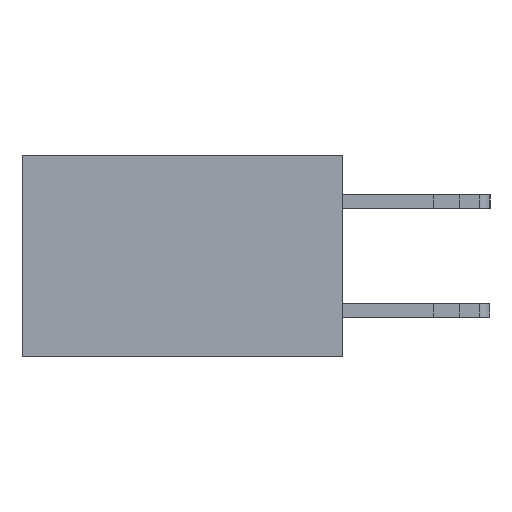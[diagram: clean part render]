
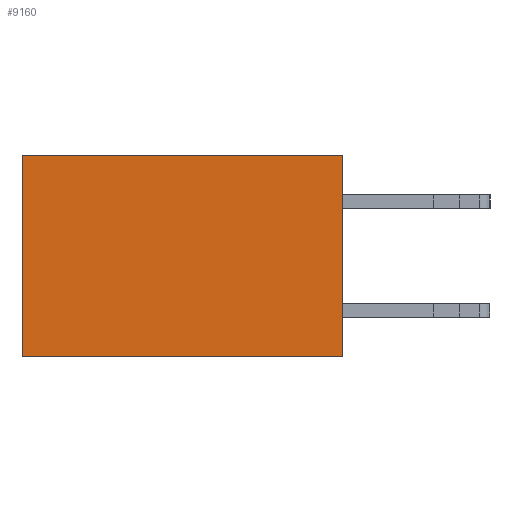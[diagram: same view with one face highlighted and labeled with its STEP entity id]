
A CAD part, left-side view. The second image highlights one B-rep face of the part: STEP entity #9160.
In plain terms, the highlighted planar face has unit normal (-1, 0, 0).
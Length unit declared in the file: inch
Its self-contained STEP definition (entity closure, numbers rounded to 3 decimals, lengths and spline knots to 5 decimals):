
#877 = VERTEX_POINT ( 'NONE', #22415 ) ;
#1611 = ORIENTED_EDGE ( 'NONE', *, *, #1914, .T. ) ;
#1914 = EDGE_CURVE ( 'NONE', #23389, #8918, #18854, .T. ) ;
#2742 = CARTESIAN_POINT ( 'NONE',  ( 0.277, 0., -0.37 ) ) ;
#3671 = DIRECTION ( 'NONE',  ( 0., 0., -1. ) ) ;
#3804 = VECTOR ( 'NONE', #12381, 39.37008 ) ;
#4152 = CARTESIAN_POINT ( 'NONE',  ( 0.277, 0., -0.37 ) ) ;
#6140 = DIRECTION ( 'NONE',  ( 0., 1., 0. ) ) ;
#6161 = VERTEX_POINT ( 'NONE', #11877 ) ;
#6810 = EDGE_LOOP ( 'NONE', ( #1611, #12000, #22275, #7375 ) ) ;
#7375 = ORIENTED_EDGE ( 'NONE', *, *, #15872, .T. ) ;
#7888 = DIRECTION ( 'NONE',  ( 0., 0., -1. ) ) ;
#8499 = VECTOR ( 'NONE', #7888, 39.37008 ) ;
#8918 = VERTEX_POINT ( 'NONE', #22404 ) ;
#9160 = ADVANCED_FACE ( 'NONE', ( #15020 ), #15302, .F. ) ;
#9585 = LINE ( 'NONE', #2742, #19305 ) ;
#9665 = VECTOR ( 'NONE', #6140, 39.37008 ) ;
#10373 = CARTESIAN_POINT ( 'NONE',  ( 0.277, 0., 0. ) ) ;
#11195 = EDGE_CURVE ( 'NONE', #6161, #877, #9585, .T. ) ;
#11877 = CARTESIAN_POINT ( 'NONE',  ( 0.277, 0., 0. ) ) ;
#12000 = ORIENTED_EDGE ( 'NONE', *, *, #19004, .F. ) ;
#12381 = DIRECTION ( 'NONE',  ( 0., 1., 0. ) ) ;
#13451 = CARTESIAN_POINT ( 'NONE',  ( 0.277, 0., -0.37 ) ) ;
#14214 = LINE ( 'NONE', #10373, #3804 ) ;
#14872 = LINE ( 'NONE', #4152, #9665 ) ;
#15020 = FACE_OUTER_BOUND ( 'NONE', #6810, .T. ) ;
#15302 = PLANE ( 'NONE',  #22919 ) ;
#15387 = DIRECTION ( 'NONE',  ( 1., 0., 0. ) ) ;
#15872 = EDGE_CURVE ( 'NONE', #6161, #23389, #14214, .T. ) ;
#16407 = DIRECTION ( 'NONE',  ( 0., 0., -1. ) ) ;
#16441 = CARTESIAN_POINT ( 'NONE',  ( 0.277, 0.59, 0. ) ) ;
#18854 = LINE ( 'NONE', #22325, #8499 ) ;
#19004 = EDGE_CURVE ( 'NONE', #877, #8918, #14872, .T. ) ;
#19305 = VECTOR ( 'NONE', #16407, 39.37008 ) ;
#22275 = ORIENTED_EDGE ( 'NONE', *, *, #11195, .F. ) ;
#22325 = CARTESIAN_POINT ( 'NONE',  ( 0.277, 0.59, -0.37 ) ) ;
#22404 = CARTESIAN_POINT ( 'NONE',  ( 0.277, 0.59, -0.37 ) ) ;
#22415 = CARTESIAN_POINT ( 'NONE',  ( 0.277, 0., -0.37 ) ) ;
#22919 = AXIS2_PLACEMENT_3D ( 'NONE', #13451, #15387, #3671 ) ;
#23389 = VERTEX_POINT ( 'NONE', #16441 ) ;
